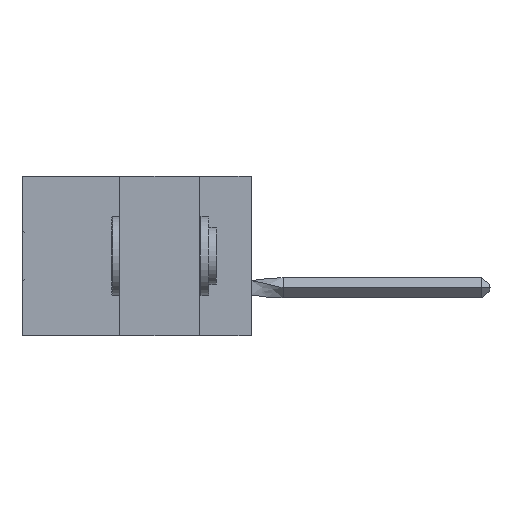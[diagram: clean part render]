
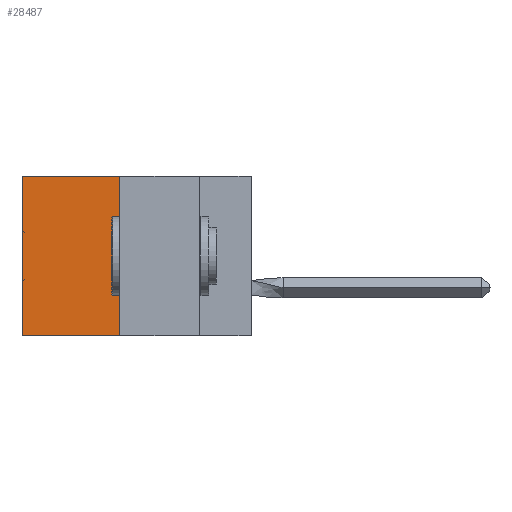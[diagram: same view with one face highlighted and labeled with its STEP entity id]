
A CAD part, left-side view. The second image highlights one B-rep face of the part: STEP entity #28487.
In plain terms, the highlighted planar face has unit normal (-1, 0, 0).
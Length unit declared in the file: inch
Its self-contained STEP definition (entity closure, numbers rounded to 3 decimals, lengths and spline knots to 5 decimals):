
#956 = CARTESIAN_POINT ( 'NONE',  ( 0.305, 0.72, -0.5 ) ) ;
#5289 = CARTESIAN_POINT ( 'NONE',  ( 0.305, 0.413, 0. ) ) ;
#5432 = VERTEX_POINT ( 'NONE', #49589 ) ;
#6469 = EDGE_LOOP ( 'NONE', ( #30910, #17061, #35718, #43107 ) ) ;
#6964 = VECTOR ( 'NONE', #40240, 39.37008 ) ;
#8098 = VERTEX_POINT ( 'NONE', #51226 ) ;
#9732 = LINE ( 'NONE', #32574, #27011 ) ;
#10458 = DIRECTION ( 'NONE',  ( 0., 1., 0. ) ) ;
#12332 = VECTOR ( 'NONE', #10458, 39.37008 ) ;
#12529 = LINE ( 'NONE', #956, #6964 ) ;
#13302 = CARTESIAN_POINT ( 'NONE',  ( 0.305, 0.413, -0.5 ) ) ;
#14167 = LINE ( 'NONE', #38532, #12332 ) ;
#14237 = EDGE_CURVE ( 'NONE', #34760, #5432, #14167, .T. ) ;
#17061 = ORIENTED_EDGE ( 'NONE', *, *, #21134, .F. ) ;
#17609 = DIRECTION ( 'NONE',  ( 1., 0., 0. ) ) ;
#20692 = DIRECTION ( 'NONE',  ( 0., 0., -1. ) ) ;
#21134 = EDGE_CURVE ( 'NONE', #22586, #8098, #9732, .T. ) ;
#22586 = VERTEX_POINT ( 'NONE', #25582 ) ;
#25582 = CARTESIAN_POINT ( 'NONE',  ( 0.305, 0.413, -0.5 ) ) ;
#27011 = VECTOR ( 'NONE', #47670, 39.37008 ) ;
#28487 = ADVANCED_FACE ( 'NONE', ( #30828 ), #49124, .F. ) ;
#30828 = FACE_OUTER_BOUND ( 'NONE', #6469, .T. ) ;
#30910 = ORIENTED_EDGE ( 'NONE', *, *, #43157, .T. ) ;
#32574 = CARTESIAN_POINT ( 'NONE',  ( 0.305, 0.413, -0.5 ) ) ;
#34760 = VERTEX_POINT ( 'NONE', #5289 ) ;
#35718 = ORIENTED_EDGE ( 'NONE', *, *, #41745, .F. ) ;
#37640 = DIRECTION ( 'NONE',  ( 0., 0., -1. ) ) ;
#38532 = CARTESIAN_POINT ( 'NONE',  ( 0.305, 0.413, 0. ) ) ;
#40240 = DIRECTION ( 'NONE',  ( 0., 0., -1. ) ) ;
#41476 = CARTESIAN_POINT ( 'NONE',  ( 0.305, 0.413, -0.5 ) ) ;
#41745 = EDGE_CURVE ( 'NONE', #34760, #22586, #47516, .T. ) ;
#43107 = ORIENTED_EDGE ( 'NONE', *, *, #14237, .T. ) ;
#43157 = EDGE_CURVE ( 'NONE', #5432, #8098, #12529, .T. ) ;
#43818 = VECTOR ( 'NONE', #37640, 39.37008 ) ;
#45844 = AXIS2_PLACEMENT_3D ( 'NONE', #13302, #17609, #20692 ) ;
#47516 = LINE ( 'NONE', #41476, #43818 ) ;
#47670 = DIRECTION ( 'NONE',  ( 0., 1., 0. ) ) ;
#49124 = PLANE ( 'NONE',  #45844 ) ;
#49589 = CARTESIAN_POINT ( 'NONE',  ( 0.305, 0.72, 0. ) ) ;
#51226 = CARTESIAN_POINT ( 'NONE',  ( 0.305, 0.72, -0.5 ) ) ;
